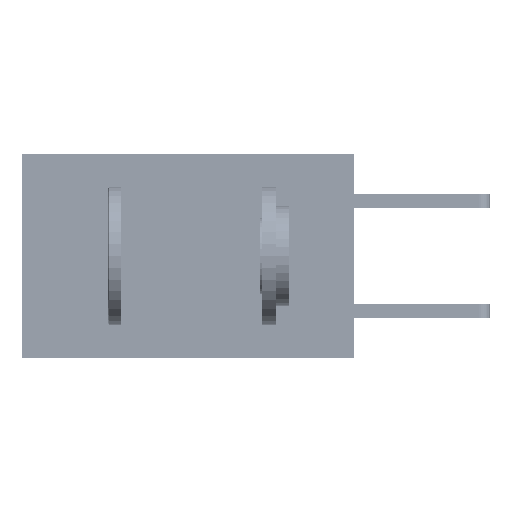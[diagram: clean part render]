
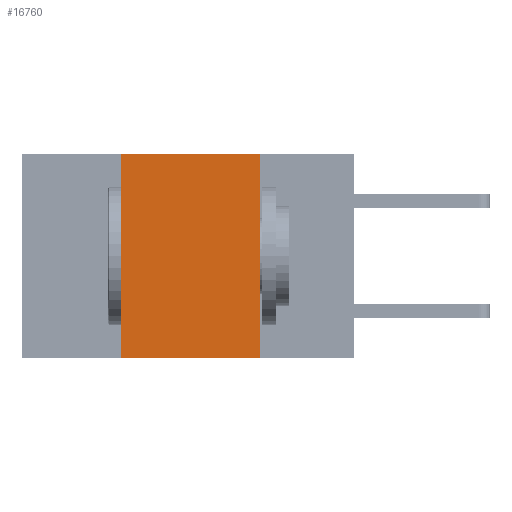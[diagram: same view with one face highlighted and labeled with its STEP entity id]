
A CAD part, left-side view. The second image highlights one B-rep face of the part: STEP entity #16760.
In plain terms, the highlighted planar face has unit normal (-1, 0, 0).
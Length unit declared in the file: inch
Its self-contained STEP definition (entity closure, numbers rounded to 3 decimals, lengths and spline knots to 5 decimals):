
#305 = LINE ( 'NONE', #36613, #16970 ) ;
#1093 = EDGE_CURVE ( 'NONE', #1661, #19257, #21477, .T. ) ;
#1262 = ORIENTED_EDGE ( 'NONE', *, *, #11194, .F. ) ;
#1661 = VERTEX_POINT ( 'NONE', #31062 ) ;
#6790 = DIRECTION ( 'NONE',  ( 0., 0., -1. ) ) ;
#7261 = ORIENTED_EDGE ( 'NONE', *, *, #8620, .F. ) ;
#7779 = FACE_OUTER_BOUND ( 'NONE', #16803, .T. ) ;
#8620 = EDGE_CURVE ( 'NONE', #36440, #32046, #10173, .T. ) ;
#9873 = CARTESIAN_POINT ( 'NONE',  ( 0., 0.17, 0. ) ) ;
#10173 = LINE ( 'NONE', #33356, #37821 ) ;
#10789 = CARTESIAN_POINT ( 'NONE',  ( 0., 0.42, 0. ) ) ;
#11194 = EDGE_CURVE ( 'NONE', #32046, #19257, #19153, .T. ) ;
#13313 = VECTOR ( 'NONE', #31493, 39.37008 ) ;
#16760 = ADVANCED_FACE ( 'NONE', ( #7779 ), #38691, .F. ) ;
#16803 = EDGE_LOOP ( 'NONE', ( #1262, #7261, #32884, #25743 ) ) ;
#16970 = VECTOR ( 'NONE', #27377, 39.37008 ) ;
#18127 = DIRECTION ( 'NONE',  ( 0., 0., -1. ) ) ;
#18509 = DIRECTION ( 'NONE',  ( 0., -1., 0. ) ) ;
#19153 = LINE ( 'NONE', #19180, #35411 ) ;
#19180 = CARTESIAN_POINT ( 'NONE',  ( 0., 0.17, 0. ) ) ;
#19257 = VERTEX_POINT ( 'NONE', #22973 ) ;
#19860 = CARTESIAN_POINT ( 'NONE',  ( 0., 0.6, -0.37 ) ) ;
#20128 = DIRECTION ( 'NONE',  ( 1., 0., 0. ) ) ;
#21477 = LINE ( 'NONE', #19860, #13313 ) ;
#22973 = CARTESIAN_POINT ( 'NONE',  ( 0., 0.17, -0.37 ) ) ;
#25743 = ORIENTED_EDGE ( 'NONE', *, *, #1093, .T. ) ;
#26479 = EDGE_CURVE ( 'NONE', #1661, #36440, #305, .T. ) ;
#27377 = DIRECTION ( 'NONE',  ( 0., 0., 1. ) ) ;
#31062 = CARTESIAN_POINT ( 'NONE',  ( 0., 0.42, -0.37 ) ) ;
#31493 = DIRECTION ( 'NONE',  ( 0., -1., 0. ) ) ;
#32046 = VERTEX_POINT ( 'NONE', #9873 ) ;
#32884 = ORIENTED_EDGE ( 'NONE', *, *, #26479, .F. ) ;
#33356 = CARTESIAN_POINT ( 'NONE',  ( 0., 0.6, 0. ) ) ;
#34912 = AXIS2_PLACEMENT_3D ( 'NONE', #38421, #20128, #18127 ) ;
#35411 = VECTOR ( 'NONE', #6790, 39.37008 ) ;
#36440 = VERTEX_POINT ( 'NONE', #10789 ) ;
#36613 = CARTESIAN_POINT ( 'NONE',  ( 0., 0.42, 0. ) ) ;
#37821 = VECTOR ( 'NONE', #18509, 39.37008 ) ;
#38421 = CARTESIAN_POINT ( 'NONE',  ( 0., 0.6, 0. ) ) ;
#38691 = PLANE ( 'NONE',  #34912 ) ;
